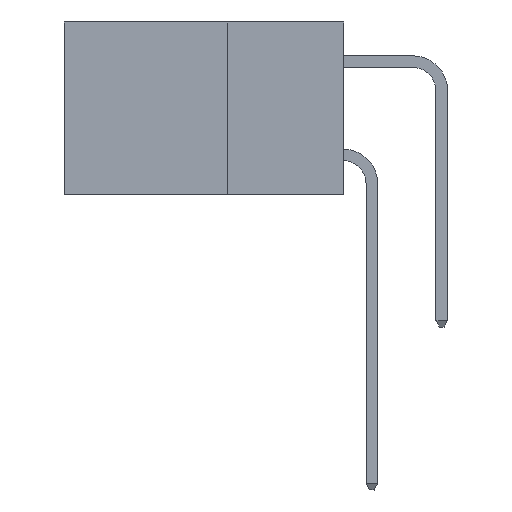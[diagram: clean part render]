
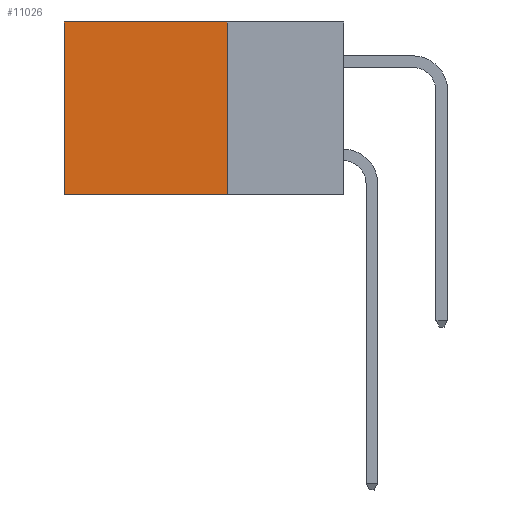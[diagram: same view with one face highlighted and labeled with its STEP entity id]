
A CAD part, left-side view. The second image highlights one B-rep face of the part: STEP entity #11026.
In plain terms, the highlighted planar face has unit normal (-1, 0, 0).
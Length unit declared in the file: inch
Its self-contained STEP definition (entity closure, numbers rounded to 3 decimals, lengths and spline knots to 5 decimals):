
#122 = PLANE ( 'NONE',  #15831 ) ;
#1293 = VECTOR ( 'NONE', #3702, 39.37008 ) ;
#1618 = DIRECTION ( 'NONE',  ( 1., 0., 0. ) ) ;
#1746 = LINE ( 'NONE', #2226, #1293 ) ;
#2226 = CARTESIAN_POINT ( 'NONE',  ( 0.298, 0.6, 0. ) ) ;
#2861 = VECTOR ( 'NONE', #16574, 39.37008 ) ;
#3702 = DIRECTION ( 'NONE',  ( 0., 0., -1. ) ) ;
#3804 = VERTEX_POINT ( 'NONE', #8375 ) ;
#3960 = CARTESIAN_POINT ( 'NONE',  ( 0.298, 0.6, -0.37 ) ) ;
#4472 = VERTEX_POINT ( 'NONE', #3960 ) ;
#5160 = CARTESIAN_POINT ( 'NONE',  ( 0.298, 0.25, 0. ) ) ;
#6270 = DIRECTION ( 'NONE',  ( 0., 1., 0. ) ) ;
#6334 = VERTEX_POINT ( 'NONE', #13200 ) ;
#7291 = ORIENTED_EDGE ( 'NONE', *, *, #16599, .F. ) ;
#7370 = VERTEX_POINT ( 'NONE', #14100 ) ;
#8027 = VECTOR ( 'NONE', #6270, 39.37008 ) ;
#8375 = CARTESIAN_POINT ( 'NONE',  ( 0.298, 0.6, 0. ) ) ;
#9019 = CARTESIAN_POINT ( 'NONE',  ( 0.298, 0.25, 0. ) ) ;
#9880 = LINE ( 'NONE', #12180, #16954 ) ;
#10673 = EDGE_CURVE ( 'NONE', #6334, #7370, #14868, .T. ) ;
#11026 = ADVANCED_FACE ( 'NONE', ( #11983 ), #122, .F. ) ;
#11875 = DIRECTION ( 'NONE',  ( 0., 0., -1. ) ) ;
#11983 = FACE_OUTER_BOUND ( 'NONE', #17270, .T. ) ;
#12180 = CARTESIAN_POINT ( 'NONE',  ( 0.298, 0.25, 0. ) ) ;
#13200 = CARTESIAN_POINT ( 'NONE',  ( 0.298, 0.25, 0. ) ) ;
#14100 = CARTESIAN_POINT ( 'NONE',  ( 0.298, 0.25, -0.37 ) ) ;
#14671 = EDGE_CURVE ( 'NONE', #6334, #3804, #9880, .T. ) ;
#14868 = LINE ( 'NONE', #5160, #2861 ) ;
#15526 = ORIENTED_EDGE ( 'NONE', *, *, #10673, .F. ) ;
#15574 = ORIENTED_EDGE ( 'NONE', *, *, #14671, .T. ) ;
#15596 = LINE ( 'NONE', #16308, #8027 ) ;
#15831 = AXIS2_PLACEMENT_3D ( 'NONE', #9019, #1618, #11875 ) ;
#16308 = CARTESIAN_POINT ( 'NONE',  ( 0.298, 0.25, -0.37 ) ) ;
#16574 = DIRECTION ( 'NONE',  ( 0., 0., -1. ) ) ;
#16599 = EDGE_CURVE ( 'NONE', #7370, #4472, #15596, .T. ) ;
#16763 = EDGE_CURVE ( 'NONE', #3804, #4472, #1746, .T. ) ;
#16954 = VECTOR ( 'NONE', #17868, 39.37008 ) ;
#17059 = ORIENTED_EDGE ( 'NONE', *, *, #16763, .T. ) ;
#17270 = EDGE_LOOP ( 'NONE', ( #17059, #7291, #15526, #15574 ) ) ;
#17868 = DIRECTION ( 'NONE',  ( 0., 1., 0. ) ) ;
